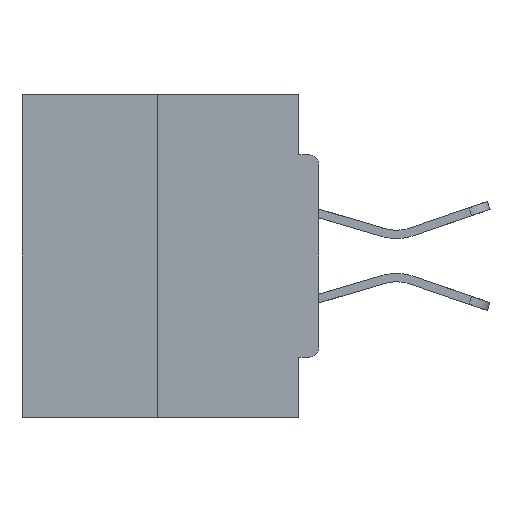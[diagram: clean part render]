
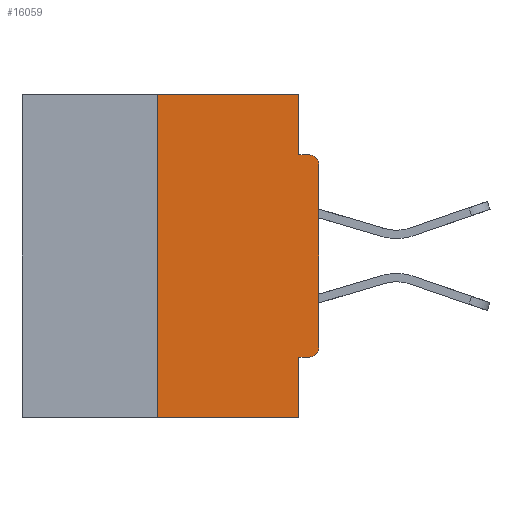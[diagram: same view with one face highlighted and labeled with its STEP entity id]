
A CAD part, left-side view. The second image highlights one B-rep face of the part: STEP entity #16059.
In plain terms, the highlighted planar face has unit normal (-1, 0, 0).
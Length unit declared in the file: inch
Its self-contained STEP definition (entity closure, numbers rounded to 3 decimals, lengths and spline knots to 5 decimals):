
#1370 = EDGE_CURVE ( 'NONE', #20880, #26267, #15989, .T. ) ;
#1450 = EDGE_CURVE ( 'NONE', #7861, #6962, #6201, .T. ) ;
#1871 = AXIS2_PLACEMENT_3D ( 'NONE', #9414, #4398, #7015 ) ;
#1970 = VECTOR ( 'NONE', #13498, 39.37008 ) ;
#2067 = DIRECTION ( 'NONE',  ( 0., 1., 0. ) ) ;
#3066 = ORIENTED_EDGE ( 'NONE', *, *, #32020, .T. ) ;
#3258 = VECTOR ( 'NONE', #11560, 39.37008 ) ;
#3407 = VECTOR ( 'NONE', #2067, 39.37008 ) ;
#3626 = ORIENTED_EDGE ( 'NONE', *, *, #27854, .F. ) ;
#3640 = VECTOR ( 'NONE', #4470, 39.37008 ) ;
#3659 = ORIENTED_EDGE ( 'NONE', *, *, #1450, .F. ) ;
#4192 = VECTOR ( 'NONE', #9377, 39.37008 ) ;
#4398 = DIRECTION ( 'NONE',  ( 1., 0., 0. ) ) ;
#4470 = DIRECTION ( 'NONE',  ( 0., -1., 0. ) ) ;
#5303 = LINE ( 'NONE', #8928, #3258 ) ;
#6201 = LINE ( 'NONE', #7310, #31112 ) ;
#6499 = VECTOR ( 'NONE', #12246, 39.37008 ) ;
#6852 = CARTESIAN_POINT ( 'NONE',  ( 0., 0.46, -0.5 ) ) ;
#6962 = VERTEX_POINT ( 'NONE', #23354 ) ;
#7015 = DIRECTION ( 'NONE',  ( 0., 0., -1. ) ) ;
#7310 = CARTESIAN_POINT ( 'NONE',  ( 0., 0.46, 0. ) ) ;
#7861 = VERTEX_POINT ( 'NONE', #9571 ) ;
#8345 = DIRECTION ( 'NONE',  ( 0., 0., -1. ) ) ;
#8385 = ORIENTED_EDGE ( 'NONE', *, *, #21462, .T. ) ;
#8552 = VERTEX_POINT ( 'NONE', #25498 ) ;
#8928 = CARTESIAN_POINT ( 'NONE',  ( 0., 0.031, 0. ) ) ;
#9265 = VERTEX_POINT ( 'NONE', #10044 ) ;
#9377 = DIRECTION ( 'NONE',  ( 0., -1., 0. ) ) ;
#9414 = CARTESIAN_POINT ( 'NONE',  ( 0., 0.46, 0. ) ) ;
#9536 = LINE ( 'NONE', #14951, #3407 ) ;
#9571 = CARTESIAN_POINT ( 'NONE',  ( 0., 0.25, 0. ) ) ;
#9602 = CARTESIAN_POINT ( 'NONE',  ( 0., 0.031, -0.5 ) ) ;
#10044 = CARTESIAN_POINT ( 'NONE',  ( 0., 0., -0.1085 ) ) ;
#10564 = VERTEX_POINT ( 'NONE', #26789 ) ;
#10623 = DIRECTION ( 'NONE',  ( -1., 0., 0. ) ) ;
#10788 = ORIENTED_EDGE ( 'NONE', *, *, #11671, .T. ) ;
#11134 = CARTESIAN_POINT ( 'NONE',  ( 0., 0., -0.3915 ) ) ;
#11560 = DIRECTION ( 'NONE',  ( 0., 0., -1. ) ) ;
#11671 = EDGE_CURVE ( 'NONE', #20182, #32195, #26773, .T. ) ;
#11907 = CARTESIAN_POINT ( 'NONE',  ( 0., 0., -0.0935 ) ) ;
#12246 = DIRECTION ( 'NONE',  ( 0., 0., -1. ) ) ;
#12906 = ORIENTED_EDGE ( 'NONE', *, *, #13803, .F. ) ;
#13074 = CARTESIAN_POINT ( 'NONE',  ( 0., 0.031, -0.4065 ) ) ;
#13498 = DIRECTION ( 'NONE',  ( 0., 0., 1. ) ) ;
#13803 = EDGE_CURVE ( 'NONE', #20182, #22750, #9536, .T. ) ;
#13840 = CIRCLE ( 'NONE', #16654, 0.015 ) ;
#14655 = PLANE ( 'NONE',  #1871 ) ;
#14951 = CARTESIAN_POINT ( 'NONE',  ( 0., 0., -0.4065 ) ) ;
#14955 = DIRECTION ( 'NONE',  ( 0., -1., 0. ) ) ;
#15485 = CARTESIAN_POINT ( 'NONE',  ( 0., 0., 0. ) ) ;
#15989 = LINE ( 'NONE', #11907, #4192 ) ;
#16059 = ADVANCED_FACE ( 'NONE', ( #28167 ), #14655, .F. ) ;
#16654 = AXIS2_PLACEMENT_3D ( 'NONE', #18364, #31499, #26137 ) ;
#17868 = DIRECTION ( 'NONE',  ( 0., 0., 1. ) ) ;
#18364 = CARTESIAN_POINT ( 'NONE',  ( 0., 0.015, -0.1085 ) ) ;
#18441 = CARTESIAN_POINT ( 'NONE',  ( 0., 0.015, -0.4065 ) ) ;
#19094 = VECTOR ( 'NONE', #17868, 39.37008 ) ;
#19548 = LINE ( 'NONE', #6852, #3640 ) ;
#20182 = VERTEX_POINT ( 'NONE', #18441 ) ;
#20880 = VERTEX_POINT ( 'NONE', #23754 ) ;
#21023 = AXIS2_PLACEMENT_3D ( 'NONE', #26262, #10623, #8345 ) ;
#21462 = EDGE_CURVE ( 'NONE', #9265, #26267, #13840, .T. ) ;
#21751 = EDGE_CURVE ( 'NONE', #10564, #8552, #19548, .T. ) ;
#22750 = VERTEX_POINT ( 'NONE', #13074 ) ;
#23153 = LINE ( 'NONE', #23413, #1970 ) ;
#23354 = CARTESIAN_POINT ( 'NONE',  ( 0., 0.031, 0. ) ) ;
#23413 = CARTESIAN_POINT ( 'NONE',  ( 0., 0.25, 0. ) ) ;
#23754 = CARTESIAN_POINT ( 'NONE',  ( 0., 0.031, -0.0935 ) ) ;
#24019 = LINE ( 'NONE', #9602, #6499 ) ;
#25498 = CARTESIAN_POINT ( 'NONE',  ( 0., 0.031, -0.5 ) ) ;
#26137 = DIRECTION ( 'NONE',  ( 0., 0., -1. ) ) ;
#26262 = CARTESIAN_POINT ( 'NONE',  ( 0., 0.015, -0.3915 ) ) ;
#26267 = VERTEX_POINT ( 'NONE', #33706 ) ;
#26773 = CIRCLE ( 'NONE', #21023, 0.015 ) ;
#26789 = CARTESIAN_POINT ( 'NONE',  ( 0., 0.25, -0.5 ) ) ;
#26900 = EDGE_LOOP ( 'NONE', ( #3659, #28519, #32855, #27233, #12906, #10788, #3066, #8385, #32155, #3626 ) ) ;
#27233 = ORIENTED_EDGE ( 'NONE', *, *, #27990, .F. ) ;
#27854 = EDGE_CURVE ( 'NONE', #6962, #20880, #5303, .T. ) ;
#27990 = EDGE_CURVE ( 'NONE', #22750, #8552, #24019, .T. ) ;
#28167 = FACE_OUTER_BOUND ( 'NONE', #26900, .T. ) ;
#28519 = ORIENTED_EDGE ( 'NONE', *, *, #33183, .F. ) ;
#29313 = LINE ( 'NONE', #15485, #19094 ) ;
#31112 = VECTOR ( 'NONE', #14955, 39.37008 ) ;
#31499 = DIRECTION ( 'NONE',  ( -1., 0., 0. ) ) ;
#32020 = EDGE_CURVE ( 'NONE', #32195, #9265, #29313, .T. ) ;
#32155 = ORIENTED_EDGE ( 'NONE', *, *, #1370, .F. ) ;
#32195 = VERTEX_POINT ( 'NONE', #11134 ) ;
#32855 = ORIENTED_EDGE ( 'NONE', *, *, #21751, .T. ) ;
#33183 = EDGE_CURVE ( 'NONE', #10564, #7861, #23153, .T. ) ;
#33706 = CARTESIAN_POINT ( 'NONE',  ( 0., 0.015, -0.0935 ) ) ;
